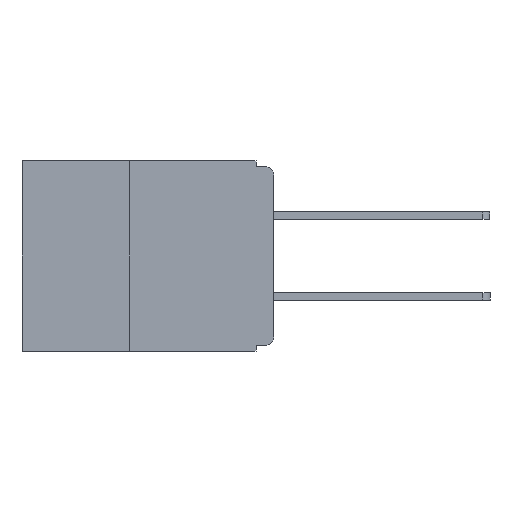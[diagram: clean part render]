
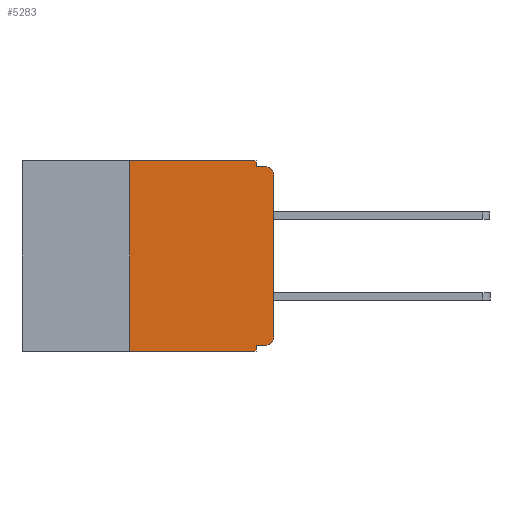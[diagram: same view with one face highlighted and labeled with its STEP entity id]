
A CAD part, left-side view. The second image highlights one B-rep face of the part: STEP entity #5283.
In plain terms, the highlighted planar face has unit normal (-1, 0, 0).
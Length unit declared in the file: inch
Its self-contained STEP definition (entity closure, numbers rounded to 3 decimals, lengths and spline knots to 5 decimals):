
#10 = ORIENTED_EDGE ( 'NONE', *, *, #4920, .F. ) ;
#20 = EDGE_CURVE ( 'NONE', #6048, #7091, #8372, .T. ) ;
#28 = CARTESIAN_POINT ( 'NONE',  ( 0., 0.015, -0.01 ) ) ;
#151 = ORIENTED_EDGE ( 'NONE', *, *, #5591, .F. ) ;
#324 = ORIENTED_EDGE ( 'NONE', *, *, #6216, .F. ) ;
#352 = CARTESIAN_POINT ( 'NONE',  ( 0., 0.031, -0.32 ) ) ;
#383 = DIRECTION ( 'NONE',  ( 0., 0., -1. ) ) ;
#514 = EDGE_CURVE ( 'NONE', #11653, #6547, #823, .T. ) ;
#524 = LINE ( 'NONE', #5900, #4508 ) ;
#554 = ORIENTED_EDGE ( 'NONE', *, *, #2447, .F. ) ;
#633 = ORIENTED_EDGE ( 'NONE', *, *, #2627, .F. ) ;
#782 = CARTESIAN_POINT ( 'NONE',  ( 0., 0., -0.305 ) ) ;
#823 = LINE ( 'NONE', #8981, #10785 ) ;
#847 = ORIENTED_EDGE ( 'NONE', *, *, #514, .T. ) ;
#900 = ORIENTED_EDGE ( 'NONE', *, *, #11382, .F. ) ;
#1019 = DIRECTION ( 'NONE',  ( -1., 0., 0. ) ) ;
#1455 = EDGE_LOOP ( 'NONE', ( #3698, #6479, #10, #151, #324, #554, #847, #900, #633, #2691 ) ) ;
#1708 = VECTOR ( 'NONE', #6454, 39.37008 ) ;
#2037 = LINE ( 'NONE', #6698, #1708 ) ;
#2156 = VECTOR ( 'NONE', #2449, 39.37008 ) ;
#2239 = EDGE_CURVE ( 'NONE', #4228, #9405, #6725, .T. ) ;
#2257 = VERTEX_POINT ( 'NONE', #352 ) ;
#2317 = VECTOR ( 'NONE', #11279, 39.37008 ) ;
#2447 = EDGE_CURVE ( 'NONE', #11653, #9050, #7446, .T. ) ;
#2449 = DIRECTION ( 'NONE',  ( 0., 0., 1. ) ) ;
#2487 = CARTESIAN_POINT ( 'NONE',  ( 0., 0.015, -0.305 ) ) ;
#2576 = VECTOR ( 'NONE', #2981, 39.37008 ) ;
#2627 = EDGE_CURVE ( 'NONE', #4228, #2257, #7592, .T. ) ;
#2647 = AXIS2_PLACEMENT_3D ( 'NONE', #11123, #11134, #11093 ) ;
#2691 = ORIENTED_EDGE ( 'NONE', *, *, #2239, .T. ) ;
#2981 = DIRECTION ( 'NONE',  ( 0., 1., 0. ) ) ;
#2994 = CARTESIAN_POINT ( 'NONE',  ( 0., 0., -0.32 ) ) ;
#3372 = CARTESIAN_POINT ( 'NONE',  ( 0., 0.031, -0.33 ) ) ;
#3448 = CARTESIAN_POINT ( 'NONE',  ( 0., 0.25, 0. ) ) ;
#3631 = AXIS2_PLACEMENT_3D ( 'NONE', #2487, #1019, #383 ) ;
#3698 = ORIENTED_EDGE ( 'NONE', *, *, #5295, .T. ) ;
#3848 = VERTEX_POINT ( 'NONE', #4848 ) ;
#4097 = VECTOR ( 'NONE', #9707, 39.37008 ) ;
#4099 = CARTESIAN_POINT ( 'NONE',  ( 0., 0.031, 0. ) ) ;
#4228 = VERTEX_POINT ( 'NONE', #5203 ) ;
#4490 = CARTESIAN_POINT ( 'NONE',  ( 0., 0.25, -0.33 ) ) ;
#4508 = VECTOR ( 'NONE', #5861, 39.37008 ) ;
#4821 = LINE ( 'NONE', #11334, #2317 ) ;
#4848 = CARTESIAN_POINT ( 'NONE',  ( 0., 0.031, -0.01 ) ) ;
#4920 = EDGE_CURVE ( 'NONE', #3848, #7091, #2037, .T. ) ;
#5203 = CARTESIAN_POINT ( 'NONE',  ( 0., 0.015, -0.32 ) ) ;
#5283 = ADVANCED_FACE ( 'NONE', ( #9796 ), #11590, .F. ) ;
#5295 = EDGE_CURVE ( 'NONE', #9405, #6048, #4821, .T. ) ;
#5591 = EDGE_CURVE ( 'NONE', #11427, #3848, #11166, .T. ) ;
#5861 = DIRECTION ( 'NONE',  ( 0., -1., 0. ) ) ;
#5900 = CARTESIAN_POINT ( 'NONE',  ( 0., 0.437, 0. ) ) ;
#6048 = VERTEX_POINT ( 'NONE', #7020 ) ;
#6216 = EDGE_CURVE ( 'NONE', #9050, #11427, #524, .T. ) ;
#6356 = LINE ( 'NONE', #8676, #8852 ) ;
#6454 = DIRECTION ( 'NONE',  ( 0., -1., 0. ) ) ;
#6479 = ORIENTED_EDGE ( 'NONE', *, *, #20, .T. ) ;
#6547 = VERTEX_POINT ( 'NONE', #3372 ) ;
#6698 = CARTESIAN_POINT ( 'NONE',  ( 0., 0., -0.01 ) ) ;
#6725 = CIRCLE ( 'NONE', #3631, 0.015 ) ;
#7020 = CARTESIAN_POINT ( 'NONE',  ( 0., 0., -0.025 ) ) ;
#7091 = VERTEX_POINT ( 'NONE', #28 ) ;
#7106 = CARTESIAN_POINT ( 'NONE',  ( 0., 0.25, -0.33 ) ) ;
#7446 = LINE ( 'NONE', #7106, #2156 ) ;
#7592 = LINE ( 'NONE', #2994, #2576 ) ;
#7972 = AXIS2_PLACEMENT_3D ( 'NONE', #11500, #11489, #11448 ) ;
#8372 = CIRCLE ( 'NONE', #2647, 0.015 ) ;
#8676 = CARTESIAN_POINT ( 'NONE',  ( 0., 0.031, -0.33 ) ) ;
#8852 = VECTOR ( 'NONE', #10463, 39.37008 ) ;
#8981 = CARTESIAN_POINT ( 'NONE',  ( 0., 0.437, -0.33 ) ) ;
#9050 = VERTEX_POINT ( 'NONE', #3448 ) ;
#9405 = VERTEX_POINT ( 'NONE', #782 ) ;
#9707 = DIRECTION ( 'NONE',  ( 0., 0., -1. ) ) ;
#9712 = CARTESIAN_POINT ( 'NONE',  ( 0., 0.031, 0. ) ) ;
#9796 = FACE_OUTER_BOUND ( 'NONE', #1455, .T. ) ;
#10423 = DIRECTION ( 'NONE',  ( 0., -1., 0. ) ) ;
#10463 = DIRECTION ( 'NONE',  ( 0., 0., -1. ) ) ;
#10785 = VECTOR ( 'NONE', #10423, 39.37008 ) ;
#11093 = DIRECTION ( 'NONE',  ( 0., 0., -1. ) ) ;
#11123 = CARTESIAN_POINT ( 'NONE',  ( 0., 0.015, -0.025 ) ) ;
#11134 = DIRECTION ( 'NONE',  ( -1., 0., 0. ) ) ;
#11166 = LINE ( 'NONE', #9712, #4097 ) ;
#11279 = DIRECTION ( 'NONE',  ( 0., 0., 1. ) ) ;
#11334 = CARTESIAN_POINT ( 'NONE',  ( 0., 0., 0. ) ) ;
#11382 = EDGE_CURVE ( 'NONE', #2257, #6547, #6356, .T. ) ;
#11427 = VERTEX_POINT ( 'NONE', #4099 ) ;
#11448 = DIRECTION ( 'NONE',  ( 0., 0., -1. ) ) ;
#11489 = DIRECTION ( 'NONE',  ( 1., 0., 0. ) ) ;
#11500 = CARTESIAN_POINT ( 'NONE',  ( 0., 0.437, 0. ) ) ;
#11590 = PLANE ( 'NONE',  #7972 ) ;
#11653 = VERTEX_POINT ( 'NONE', #4490 ) ;
